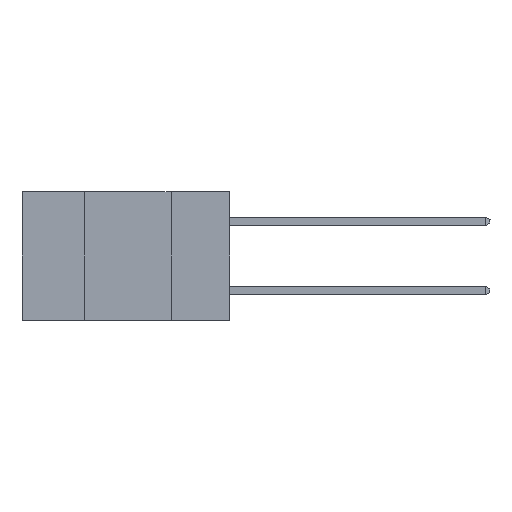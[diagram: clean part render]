
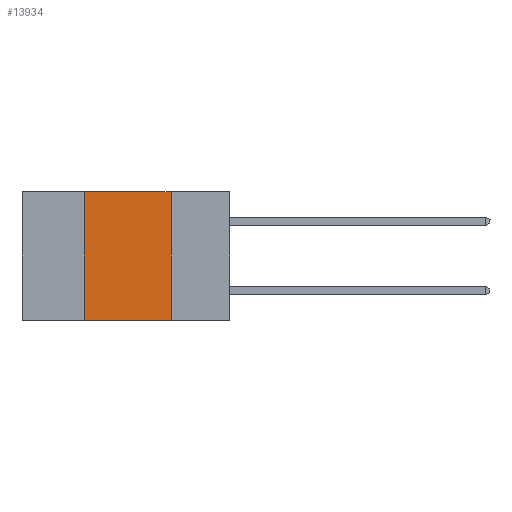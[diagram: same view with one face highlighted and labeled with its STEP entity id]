
A CAD part, left-side view. The second image highlights one B-rep face of the part: STEP entity #13934.
In plain terms, the highlighted planar face has unit normal (-1, 0, 0).
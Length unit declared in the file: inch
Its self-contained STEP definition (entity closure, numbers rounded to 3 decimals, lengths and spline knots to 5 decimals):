
#14 = VECTOR ( 'NONE', #11244, 39.37008 ) ;
#1035 = LINE ( 'NONE', #19848, #7678 ) ;
#3453 = DIRECTION ( 'NONE',  ( 0., -1., 0. ) ) ;
#7259 = DIRECTION ( 'NONE',  ( 0., -1., 0. ) ) ;
#7678 = VECTOR ( 'NONE', #7259, 39.37008 ) ;
#8344 = AXIS2_PLACEMENT_3D ( 'NONE', #22962, #12423, #25109 ) ;
#8460 = CARTESIAN_POINT ( 'NONE',  ( 0., 0.42, 0. ) ) ;
#8999 = VECTOR ( 'NONE', #24190, 39.37008 ) ;
#9257 = CARTESIAN_POINT ( 'NONE',  ( 0., 0.17, 0. ) ) ;
#9508 = VECTOR ( 'NONE', #3453, 39.37008 ) ;
#10074 = EDGE_CURVE ( 'NONE', #23137, #26244, #1035, .T. ) ;
#10473 = EDGE_CURVE ( 'NONE', #23137, #15588, #23657, .T. ) ;
#10493 = CARTESIAN_POINT ( 'NONE',  ( 0., 0.42, -0.37 ) ) ;
#11151 = LINE ( 'NONE', #16182, #9508 ) ;
#11244 = DIRECTION ( 'NONE',  ( 0., 0., 1. ) ) ;
#11299 = CARTESIAN_POINT ( 'NONE',  ( 0., 0.42, 0. ) ) ;
#12423 = DIRECTION ( 'NONE',  ( 1., 0., 0. ) ) ;
#13101 = CARTESIAN_POINT ( 'NONE',  ( 0., 0.17, -0.37 ) ) ;
#13175 = ORIENTED_EDGE ( 'NONE', *, *, #10074, .T. ) ;
#13504 = EDGE_CURVE ( 'NONE', #15588, #25733, #11151, .T. ) ;
#13934 = ADVANCED_FACE ( 'NONE', ( #16810 ), #23049, .F. ) ;
#14502 = CARTESIAN_POINT ( 'NONE',  ( 0., 0.17, 0. ) ) ;
#15588 = VERTEX_POINT ( 'NONE', #11299 ) ;
#15922 = EDGE_CURVE ( 'NONE', #25733, #26244, #27028, .T. ) ;
#16182 = CARTESIAN_POINT ( 'NONE',  ( 0., 0.6, 0. ) ) ;
#16810 = FACE_OUTER_BOUND ( 'NONE', #19022, .T. ) ;
#17000 = ORIENTED_EDGE ( 'NONE', *, *, #15922, .F. ) ;
#19022 = EDGE_LOOP ( 'NONE', ( #17000, #26976, #27313, #13175 ) ) ;
#19848 = CARTESIAN_POINT ( 'NONE',  ( 0., 0.6, -0.37 ) ) ;
#22962 = CARTESIAN_POINT ( 'NONE',  ( 0., 0.6, 0. ) ) ;
#23049 = PLANE ( 'NONE',  #8344 ) ;
#23137 = VERTEX_POINT ( 'NONE', #10493 ) ;
#23657 = LINE ( 'NONE', #8460, #14 ) ;
#24190 = DIRECTION ( 'NONE',  ( 0., 0., -1. ) ) ;
#25109 = DIRECTION ( 'NONE',  ( 0., 0., -1. ) ) ;
#25733 = VERTEX_POINT ( 'NONE', #14502 ) ;
#26244 = VERTEX_POINT ( 'NONE', #13101 ) ;
#26976 = ORIENTED_EDGE ( 'NONE', *, *, #13504, .F. ) ;
#27028 = LINE ( 'NONE', #9257, #8999 ) ;
#27313 = ORIENTED_EDGE ( 'NONE', *, *, #10473, .F. ) ;
